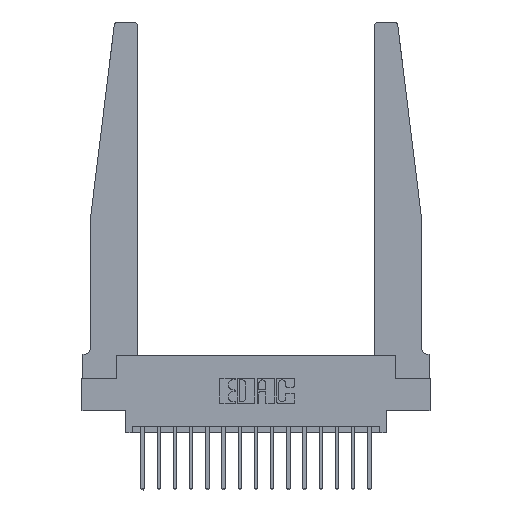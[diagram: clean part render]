
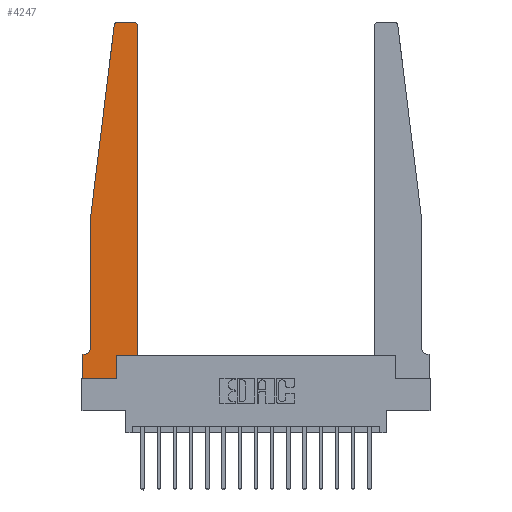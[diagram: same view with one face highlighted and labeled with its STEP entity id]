
A CAD part, top view. The second image highlights one B-rep face of the part: STEP entity #4247.
In plain terms, the highlighted planar face has unit normal (0, 0, 1).
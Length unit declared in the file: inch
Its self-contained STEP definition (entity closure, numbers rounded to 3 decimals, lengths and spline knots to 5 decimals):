
#75 = VECTOR ( 'NONE', #15755, 39.37008 ) ;
#101 = AXIS2_PLACEMENT_3D ( 'NONE', #3086, #14454, #5962 ) ;
#142 = CARTESIAN_POINT ( 'NONE',  ( 0.065, 1.25, 0.37 ) ) ;
#151 = CARTESIAN_POINT ( 'NONE',  ( 0.425, 0.18, 0.37 ) ) ;
#386 = ORIENTED_EDGE ( 'NONE', *, *, #14498, .T. ) ;
#1154 = CARTESIAN_POINT ( 'NONE',  ( 0., 0., 0.37 ) ) ;
#1237 = CARTESIAN_POINT ( 'NONE',  ( 0.425, 0.18, 0.37 ) ) ;
#1303 = DIRECTION ( 'NONE',  ( 0., 1., 0. ) ) ;
#1529 = EDGE_CURVE ( 'NONE', #8833, #4914, #10068, .T. ) ;
#1559 = LINE ( 'NONE', #8800, #16186 ) ;
#1578 = DIRECTION ( 'NONE',  ( 1., 0., 0. ) ) ;
#1636 = DIRECTION ( 'NONE',  ( 0., 0., 1. ) ) ;
#1685 = CARTESIAN_POINT ( 'NONE',  ( 0., 0., 0.37 ) ) ;
#1893 = LINE ( 'NONE', #2626, #16531 ) ;
#2106 = LINE ( 'NONE', #1237, #8793 ) ;
#2340 = ORIENTED_EDGE ( 'NONE', *, *, #7398, .T. ) ;
#2565 = CARTESIAN_POINT ( 'NONE',  ( 0.065, 1.25, 0.37 ) ) ;
#2589 = AXIS2_PLACEMENT_3D ( 'NONE', #10167, #1636, #11594 ) ;
#2626 = CARTESIAN_POINT ( 'NONE',  ( 0.065, 1.25, 0.37 ) ) ;
#3069 = EDGE_CURVE ( 'NONE', #11568, #9946, #1893, .T. ) ;
#3086 = CARTESIAN_POINT ( 'NONE',  ( 0., 0.1875, 0.37 ) ) ;
#3104 = DIRECTION ( 'NONE',  ( 1., 0., 0. ) ) ;
#3676 = EDGE_CURVE ( 'NONE', #7975, #8833, #14313, .T. ) ;
#3831 = LINE ( 'NONE', #142, #75 ) ;
#4072 = EDGE_CURVE ( 'NONE', #17087, #4878, #2106, .T. ) ;
#4247 = ADVANCED_FACE ( 'NONE', ( #14097 ), #11631, .T. ) ;
#4286 = VERTEX_POINT ( 'NONE', #13121 ) ;
#4303 = ORIENTED_EDGE ( 'NONE', *, *, #8901, .T. ) ;
#4595 = VECTOR ( 'NONE', #14148, 39.37008 ) ;
#4878 = VERTEX_POINT ( 'NONE', #15773 ) ;
#4914 = VERTEX_POINT ( 'NONE', #14431 ) ;
#5031 = LINE ( 'NONE', #9958, #4595 ) ;
#5237 = CARTESIAN_POINT ( 'NONE',  ( 0.015, 0.2375, 0.37 ) ) ;
#5381 = EDGE_CURVE ( 'NONE', #9946, #12104, #3831, .T. ) ;
#5498 = CARTESIAN_POINT ( 'NONE',  ( 0.27653, 2.75, 0.37 ) ) ;
#5664 = EDGE_LOOP ( 'NONE', ( #9283, #13763, #15260, #16166, #386, #8558, #16387, #7965, #14415, #4303, #15460, #2340 ) ) ;
#5730 = VECTOR ( 'NONE', #1578, 39.37008 ) ;
#5781 = CARTESIAN_POINT ( 'NONE',  ( 0., 0., 0.37 ) ) ;
#5962 = DIRECTION ( 'NONE',  ( 1., 0., 0. ) ) ;
#6008 = DIRECTION ( 'NONE',  ( -1., 0., 0. ) ) ;
#6261 = VERTEX_POINT ( 'NONE', #11067 ) ;
#6276 = VECTOR ( 'NONE', #10369, 39.37008 ) ;
#6377 = DIRECTION ( 'NONE',  ( 0., 0., 1. ) ) ;
#6618 = AXIS2_PLACEMENT_3D ( 'NONE', #14855, #6377, #16269 ) ;
#6661 = CIRCLE ( 'NONE', #2589, 0.03 ) ;
#6672 = DIRECTION ( 'NONE',  ( -1., 0., 0. ) ) ;
#7398 = EDGE_CURVE ( 'NONE', #4878, #9238, #6661, .T. ) ;
#7502 = CARTESIAN_POINT ( 'NONE',  ( 0.2605, 0.18, 0.37 ) ) ;
#7606 = CIRCLE ( 'NONE', #17990, 0.05 ) ;
#7965 = ORIENTED_EDGE ( 'NONE', *, *, #3676, .T. ) ;
#7975 = VERTEX_POINT ( 'NONE', #5781 ) ;
#8291 = DIRECTION ( 'NONE',  ( -0.122, -0.992, 0. ) ) ;
#8558 = ORIENTED_EDGE ( 'NONE', *, *, #11285, .T. ) ;
#8793 = VECTOR ( 'NONE', #1303, 39.37008 ) ;
#8800 = CARTESIAN_POINT ( 'NONE',  ( 0.25, 2.75, 0.37 ) ) ;
#8833 = VERTEX_POINT ( 'NONE', #9916 ) ;
#8901 = EDGE_CURVE ( 'NONE', #4914, #17087, #9500, .T. ) ;
#9238 = VERTEX_POINT ( 'NONE', #12575 ) ;
#9283 = ORIENTED_EDGE ( 'NONE', *, *, #15590, .T. ) ;
#9500 = LINE ( 'NONE', #151, #5730 ) ;
#9916 = CARTESIAN_POINT ( 'NONE',  ( 0.2605, 0., 0.37 ) ) ;
#9946 = VERTEX_POINT ( 'NONE', #2565 ) ;
#9958 = CARTESIAN_POINT ( 'NONE',  ( 0.065, 0.1875, 0.37 ) ) ;
#10068 = LINE ( 'NONE', #7502, #6276 ) ;
#10167 = CARTESIAN_POINT ( 'NONE',  ( 0.395, 2.72, 0.37 ) ) ;
#10369 = DIRECTION ( 'NONE',  ( 0., 1., 0. ) ) ;
#10588 = VERTEX_POINT ( 'NONE', #5498 ) ;
#11067 = CARTESIAN_POINT ( 'NONE',  ( 0., 0.1875, 0.37 ) ) ;
#11285 = EDGE_CURVE ( 'NONE', #4286, #6261, #5031, .T. ) ;
#11423 = LINE ( 'NONE', #1154, #15584 ) ;
#11568 = VERTEX_POINT ( 'NONE', #13306 ) ;
#11594 = DIRECTION ( 'NONE',  ( 1., 0., 0. ) ) ;
#11631 = PLANE ( 'NONE',  #101 ) ;
#12104 = VERTEX_POINT ( 'NONE', #16710 ) ;
#12488 = DIRECTION ( 'NONE',  ( 0., -1., 0. ) ) ;
#12575 = CARTESIAN_POINT ( 'NONE',  ( 0.395, 2.75, 0.37 ) ) ;
#13121 = CARTESIAN_POINT ( 'NONE',  ( 0.015, 0.1875, 0.37 ) ) ;
#13306 = CARTESIAN_POINT ( 'NONE',  ( 0.24675, 2.72367, 0.37 ) ) ;
#13763 = ORIENTED_EDGE ( 'NONE', *, *, #14365, .T. ) ;
#13949 = CARTESIAN_POINT ( 'NONE',  ( 0.425, 0.18, 0.37 ) ) ;
#13951 = EDGE_CURVE ( 'NONE', #6261, #7975, #11423, .T. ) ;
#14097 = FACE_OUTER_BOUND ( 'NONE', #5664, .T. ) ;
#14148 = DIRECTION ( 'NONE',  ( -1., 0., 0. ) ) ;
#14313 = LINE ( 'NONE', #1685, #14750 ) ;
#14365 = EDGE_CURVE ( 'NONE', #10588, #11568, #16885, .T. ) ;
#14415 = ORIENTED_EDGE ( 'NONE', *, *, #1529, .T. ) ;
#14431 = CARTESIAN_POINT ( 'NONE',  ( 0.2605, 0.18, 0.37 ) ) ;
#14454 = DIRECTION ( 'NONE',  ( 0., 0., 1. ) ) ;
#14498 = EDGE_CURVE ( 'NONE', #12104, #4286, #7606, .T. ) ;
#14750 = VECTOR ( 'NONE', #3104, 39.37008 ) ;
#14855 = CARTESIAN_POINT ( 'NONE',  ( 0.27653, 2.72, 0.37 ) ) ;
#15155 = DIRECTION ( 'NONE',  ( 0., 0., -1. ) ) ;
#15260 = ORIENTED_EDGE ( 'NONE', *, *, #3069, .T. ) ;
#15460 = ORIENTED_EDGE ( 'NONE', *, *, #4072, .T. ) ;
#15584 = VECTOR ( 'NONE', #12488, 39.37008 ) ;
#15590 = EDGE_CURVE ( 'NONE', #9238, #10588, #1559, .T. ) ;
#15755 = DIRECTION ( 'NONE',  ( 0., -1., 0. ) ) ;
#15773 = CARTESIAN_POINT ( 'NONE',  ( 0.425, 2.72, 0.37 ) ) ;
#16166 = ORIENTED_EDGE ( 'NONE', *, *, #5381, .T. ) ;
#16186 = VECTOR ( 'NONE', #6008, 39.37008 ) ;
#16269 = DIRECTION ( 'NONE',  ( 1., 0., 0. ) ) ;
#16387 = ORIENTED_EDGE ( 'NONE', *, *, #13951, .T. ) ;
#16531 = VECTOR ( 'NONE', #8291, 39.37008 ) ;
#16710 = CARTESIAN_POINT ( 'NONE',  ( 0.065, 0.2375, 0.37 ) ) ;
#16885 = CIRCLE ( 'NONE', #6618, 0.03 ) ;
#17087 = VERTEX_POINT ( 'NONE', #13949 ) ;
#17990 = AXIS2_PLACEMENT_3D ( 'NONE', #5237, #15155, #6672 ) ;
